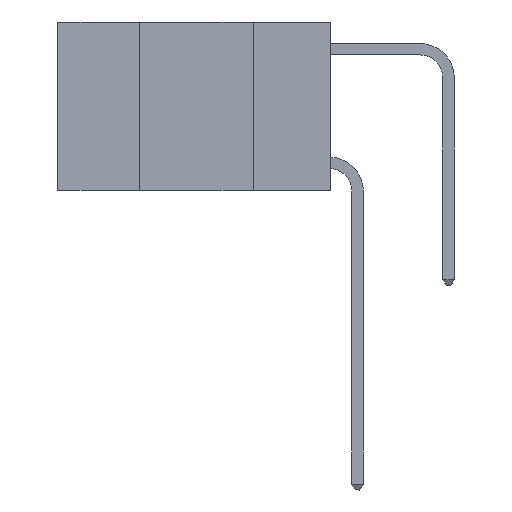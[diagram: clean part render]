
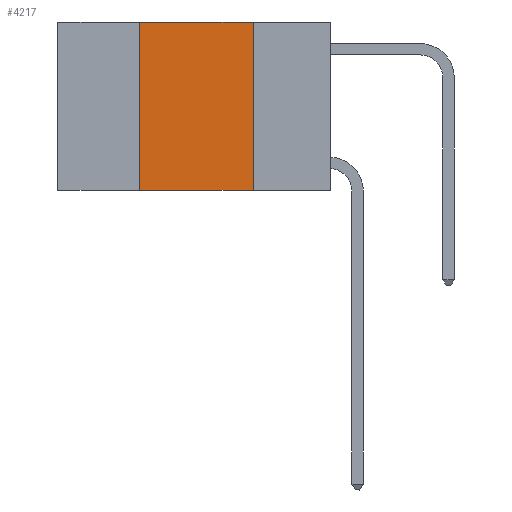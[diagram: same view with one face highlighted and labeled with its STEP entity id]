
A CAD part, left-side view. The second image highlights one B-rep face of the part: STEP entity #4217.
In plain terms, the highlighted planar face has unit normal (-1, 0, 0).
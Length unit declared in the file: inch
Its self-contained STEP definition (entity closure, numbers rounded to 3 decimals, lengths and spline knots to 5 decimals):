
#1084 = EDGE_CURVE ( 'NONE', #7327, #6799, #14208, .T. ) ;
#1676 = CARTESIAN_POINT ( 'NONE',  ( 0., 0.17, -0.37 ) ) ;
#1949 = DIRECTION ( 'NONE',  ( 0., -1., 0. ) ) ;
#1976 = ORIENTED_EDGE ( 'NONE', *, *, #5742, .F. ) ;
#2225 = VECTOR ( 'NONE', #4322, 39.37008 ) ;
#2240 = EDGE_CURVE ( 'NONE', #7327, #9204, #2421, .T. ) ;
#2421 = LINE ( 'NONE', #14755, #2225 ) ;
#2484 = VECTOR ( 'NONE', #10754, 39.37008 ) ;
#3176 = ORIENTED_EDGE ( 'NONE', *, *, #1084, .T. ) ;
#3244 = CARTESIAN_POINT ( 'NONE',  ( 0., 0.6, 0. ) ) ;
#4217 = ADVANCED_FACE ( 'NONE', ( #8490 ), #5351, .F. ) ;
#4322 = DIRECTION ( 'NONE',  ( 0., 0., 1. ) ) ;
#4420 = AXIS2_PLACEMENT_3D ( 'NONE', #8574, #10952, #14407 ) ;
#5351 = PLANE ( 'NONE',  #4420 ) ;
#5505 = CARTESIAN_POINT ( 'NONE',  ( 0., 0.6, -0.37 ) ) ;
#5556 = LINE ( 'NONE', #13756, #2484 ) ;
#5671 = CARTESIAN_POINT ( 'NONE',  ( 0., 0.42, 0. ) ) ;
#5742 = EDGE_CURVE ( 'NONE', #9204, #7787, #13416, .T. ) ;
#5814 = EDGE_LOOP ( 'NONE', ( #11310, #1976, #10358, #3176 ) ) ;
#6799 = VERTEX_POINT ( 'NONE', #1676 ) ;
#7327 = VERTEX_POINT ( 'NONE', #9662 ) ;
#7787 = VERTEX_POINT ( 'NONE', #13213 ) ;
#8490 = FACE_OUTER_BOUND ( 'NONE', #5814, .T. ) ;
#8574 = CARTESIAN_POINT ( 'NONE',  ( 0., 0.6, 0. ) ) ;
#9204 = VERTEX_POINT ( 'NONE', #5671 ) ;
#9662 = CARTESIAN_POINT ( 'NONE',  ( 0., 0.42, -0.37 ) ) ;
#10358 = ORIENTED_EDGE ( 'NONE', *, *, #2240, .F. ) ;
#10754 = DIRECTION ( 'NONE',  ( 0., 0., -1. ) ) ;
#10952 = DIRECTION ( 'NONE',  ( 1., 0., 0. ) ) ;
#11310 = ORIENTED_EDGE ( 'NONE', *, *, #14731, .F. ) ;
#12922 = VECTOR ( 'NONE', #14751, 39.37008 ) ;
#13213 = CARTESIAN_POINT ( 'NONE',  ( 0., 0.17, 0. ) ) ;
#13416 = LINE ( 'NONE', #3244, #13598 ) ;
#13598 = VECTOR ( 'NONE', #1949, 39.37008 ) ;
#13756 = CARTESIAN_POINT ( 'NONE',  ( 0., 0.17, 0. ) ) ;
#14208 = LINE ( 'NONE', #5505, #12922 ) ;
#14407 = DIRECTION ( 'NONE',  ( 0., 0., -1. ) ) ;
#14731 = EDGE_CURVE ( 'NONE', #7787, #6799, #5556, .T. ) ;
#14751 = DIRECTION ( 'NONE',  ( 0., -1., 0. ) ) ;
#14755 = CARTESIAN_POINT ( 'NONE',  ( 0., 0.42, 0. ) ) ;
